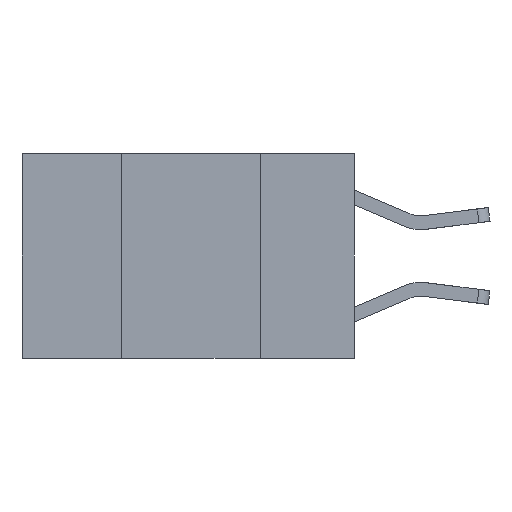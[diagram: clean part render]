
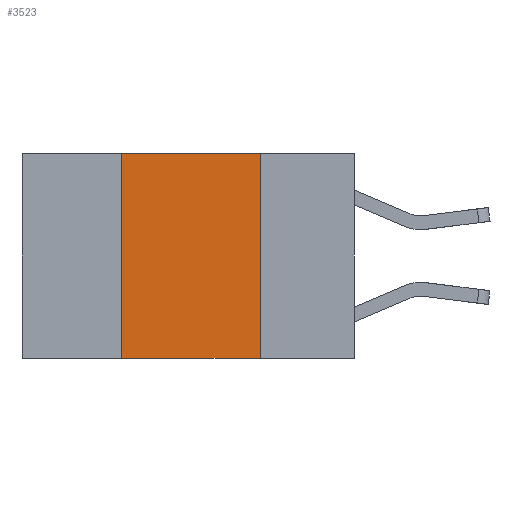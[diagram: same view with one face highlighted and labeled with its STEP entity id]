
A CAD part, left-side view. The second image highlights one B-rep face of the part: STEP entity #3523.
In plain terms, the highlighted planar face has unit normal (-1, 0, 0).
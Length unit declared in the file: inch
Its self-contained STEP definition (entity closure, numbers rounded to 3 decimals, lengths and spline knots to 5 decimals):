
#595 = CARTESIAN_POINT ( 'NONE',  ( 0., 0.17, -0.37 ) ) ;
#722 = CARTESIAN_POINT ( 'NONE',  ( 0., 0.17, 0. ) ) ;
#1495 = DIRECTION ( 'NONE',  ( 0., 0., -1. ) ) ;
#1496 = VERTEX_POINT ( 'NONE', #8016 ) ;
#1601 = DIRECTION ( 'NONE',  ( 1., 0., 0. ) ) ;
#2467 = DIRECTION ( 'NONE',  ( 0., 0., 1. ) ) ;
#2765 = EDGE_CURVE ( 'NONE', #1496, #3280, #4760, .T. ) ;
#3228 = VECTOR ( 'NONE', #1495, 39.37008 ) ;
#3280 = VERTEX_POINT ( 'NONE', #3772 ) ;
#3502 = VERTEX_POINT ( 'NONE', #5044 ) ;
#3523 = ADVANCED_FACE ( 'NONE', ( #6660 ), #9868, .F. ) ;
#3769 = CARTESIAN_POINT ( 'NONE',  ( 0., 0.6, 0. ) ) ;
#3772 = CARTESIAN_POINT ( 'NONE',  ( 0., 0.42, 0. ) ) ;
#3932 = ORIENTED_EDGE ( 'NONE', *, *, #2765, .F. ) ;
#4137 = EDGE_CURVE ( 'NONE', #1496, #4148, #4465, .T. ) ;
#4148 = VERTEX_POINT ( 'NONE', #595 ) ;
#4465 = LINE ( 'NONE', #4507, #7162 ) ;
#4495 = ORIENTED_EDGE ( 'NONE', *, *, #7971, .F. ) ;
#4507 = CARTESIAN_POINT ( 'NONE',  ( 0., 0.6, -0.37 ) ) ;
#4760 = LINE ( 'NONE', #6169, #5090 ) ;
#4786 = AXIS2_PLACEMENT_3D ( 'NONE', #8510, #1601, #6815 ) ;
#4806 = VECTOR ( 'NONE', #7700, 39.37008 ) ;
#5044 = CARTESIAN_POINT ( 'NONE',  ( 0., 0.17, 0. ) ) ;
#5090 = VECTOR ( 'NONE', #2467, 39.37008 ) ;
#6169 = CARTESIAN_POINT ( 'NONE',  ( 0., 0.42, 0. ) ) ;
#6373 = EDGE_LOOP ( 'NONE', ( #7853, #4495, #3932, #7342 ) ) ;
#6427 = EDGE_CURVE ( 'NONE', #3502, #4148, #7806, .T. ) ;
#6660 = FACE_OUTER_BOUND ( 'NONE', #6373, .T. ) ;
#6815 = DIRECTION ( 'NONE',  ( 0., 0., -1. ) ) ;
#7162 = VECTOR ( 'NONE', #8927, 39.37008 ) ;
#7342 = ORIENTED_EDGE ( 'NONE', *, *, #4137, .T. ) ;
#7650 = LINE ( 'NONE', #3769, #4806 ) ;
#7700 = DIRECTION ( 'NONE',  ( 0., -1., 0. ) ) ;
#7806 = LINE ( 'NONE', #722, #3228 ) ;
#7853 = ORIENTED_EDGE ( 'NONE', *, *, #6427, .F. ) ;
#7971 = EDGE_CURVE ( 'NONE', #3280, #3502, #7650, .T. ) ;
#8016 = CARTESIAN_POINT ( 'NONE',  ( 0., 0.42, -0.37 ) ) ;
#8510 = CARTESIAN_POINT ( 'NONE',  ( 0., 0.6, 0. ) ) ;
#8927 = DIRECTION ( 'NONE',  ( 0., -1., 0. ) ) ;
#9868 = PLANE ( 'NONE',  #4786 ) ;
